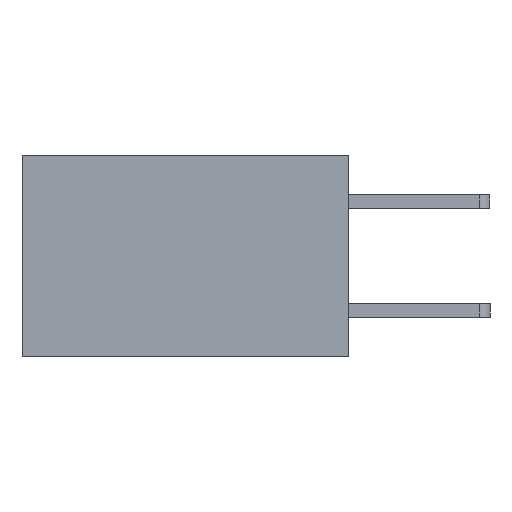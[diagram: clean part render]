
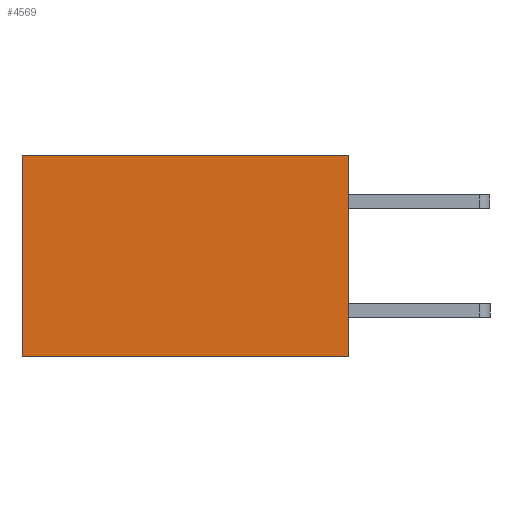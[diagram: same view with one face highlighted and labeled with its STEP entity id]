
A CAD part, left-side view. The second image highlights one B-rep face of the part: STEP entity #4569.
In plain terms, the highlighted planar face has unit normal (-1, 0, 0).
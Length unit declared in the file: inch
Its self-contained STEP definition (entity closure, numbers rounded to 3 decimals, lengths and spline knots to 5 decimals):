
#2 = CARTESIAN_POINT ( 'NONE',  ( 0.2615, 0., -0.37 ) ) ;
#94 = CARTESIAN_POINT ( 'NONE',  ( 0.2615, 0., -0.37 ) ) ;
#413 = LINE ( 'NONE', #997, #7809 ) ;
#697 = VERTEX_POINT ( 'NONE', #6170 ) ;
#699 = DIRECTION ( 'NONE',  ( 0., 0., -1. ) ) ;
#844 = EDGE_CURVE ( 'NONE', #697, #5892, #4491, .T. ) ;
#997 = CARTESIAN_POINT ( 'NONE',  ( 0.2615, 0., -0.37 ) ) ;
#1528 = DIRECTION ( 'NONE',  ( 0., 0., -1. ) ) ;
#1530 = EDGE_CURVE ( 'NONE', #5076, #2798, #3924, .T. ) ;
#1637 = CARTESIAN_POINT ( 'NONE',  ( 0.2615, 0., -0.37 ) ) ;
#2097 = PLANE ( 'NONE',  #7351 ) ;
#2412 = VECTOR ( 'NONE', #3581, 39.37008 ) ;
#2506 = VECTOR ( 'NONE', #1528, 39.37008 ) ;
#2538 = ORIENTED_EDGE ( 'NONE', *, *, #1530, .F. ) ;
#2777 = ORIENTED_EDGE ( 'NONE', *, *, #3507, .T. ) ;
#2798 = VERTEX_POINT ( 'NONE', #94 ) ;
#2993 = EDGE_CURVE ( 'NONE', #2798, #5892, #413, .T. ) ;
#3507 = EDGE_CURVE ( 'NONE', #5076, #697, #5612, .T. ) ;
#3581 = DIRECTION ( 'NONE',  ( 0., 0., -1. ) ) ;
#3924 = LINE ( 'NONE', #1637, #2506 ) ;
#4451 = CARTESIAN_POINT ( 'NONE',  ( 0.2615, 0., 0. ) ) ;
#4491 = LINE ( 'NONE', #5120, #2412 ) ;
#4518 = ORIENTED_EDGE ( 'NONE', *, *, #2993, .F. ) ;
#4569 = ADVANCED_FACE ( 'NONE', ( #6168 ), #2097, .F. ) ;
#4893 = DIRECTION ( 'NONE',  ( 1., 0., 0. ) ) ;
#5076 = VERTEX_POINT ( 'NONE', #8479 ) ;
#5120 = CARTESIAN_POINT ( 'NONE',  ( 0.2615, 0.6, -0.37 ) ) ;
#5612 = LINE ( 'NONE', #4451, #7330 ) ;
#5892 = VERTEX_POINT ( 'NONE', #8489 ) ;
#6168 = FACE_OUTER_BOUND ( 'NONE', #6169, .T. ) ;
#6169 = EDGE_LOOP ( 'NONE', ( #6613, #4518, #2538, #2777 ) ) ;
#6170 = CARTESIAN_POINT ( 'NONE',  ( 0.2615, 0.6, 0. ) ) ;
#6613 = ORIENTED_EDGE ( 'NONE', *, *, #844, .T. ) ;
#7330 = VECTOR ( 'NONE', #8101, 39.37008 ) ;
#7351 = AXIS2_PLACEMENT_3D ( 'NONE', #2, #4893, #699 ) ;
#7809 = VECTOR ( 'NONE', #8893, 39.37008 ) ;
#8101 = DIRECTION ( 'NONE',  ( 0., 1., 0. ) ) ;
#8479 = CARTESIAN_POINT ( 'NONE',  ( 0.2615, 0., 0. ) ) ;
#8489 = CARTESIAN_POINT ( 'NONE',  ( 0.2615, 0.6, -0.37 ) ) ;
#8893 = DIRECTION ( 'NONE',  ( 0., 1., 0. ) ) ;
